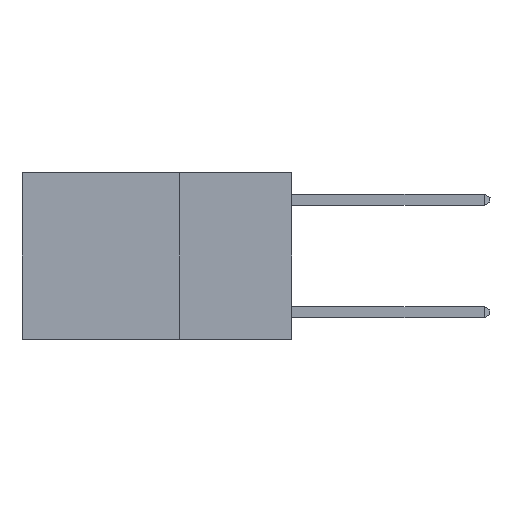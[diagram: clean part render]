
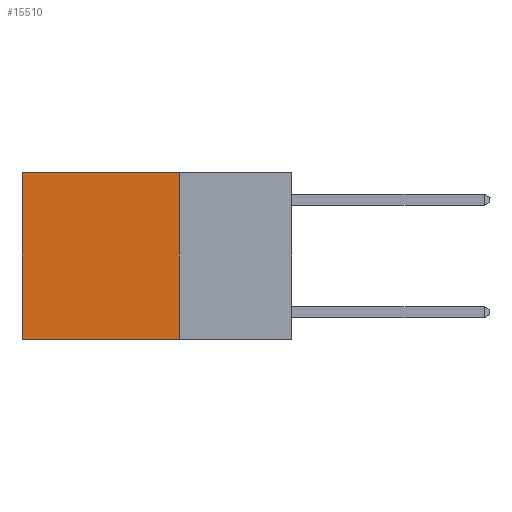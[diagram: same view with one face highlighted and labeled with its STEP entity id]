
A CAD part, left-side view. The second image highlights one B-rep face of the part: STEP entity #15510.
In plain terms, the highlighted planar face has unit normal (-1, 0, 0).
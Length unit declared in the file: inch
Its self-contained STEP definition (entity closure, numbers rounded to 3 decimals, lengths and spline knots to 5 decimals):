
#1141 = VECTOR ( 'NONE', #3060, 39.37008 ) ;
#2734 = CARTESIAN_POINT ( 'NONE',  ( 0.2625, 0.25, 0. ) ) ;
#3060 = DIRECTION ( 'NONE',  ( 0., 0., -1. ) ) ;
#3104 = ORIENTED_EDGE ( 'NONE', *, *, #19769, .T. ) ;
#3151 = CARTESIAN_POINT ( 'NONE',  ( 0.2625, 0.6, 0. ) ) ;
#4069 = CARTESIAN_POINT ( 'NONE',  ( 0.2625, 0.6, -0.37 ) ) ;
#4252 = VERTEX_POINT ( 'NONE', #4069 ) ;
#4399 = CARTESIAN_POINT ( 'NONE',  ( 0.2625, 0.6, 0. ) ) ;
#5651 = DIRECTION ( 'NONE',  ( 0., 1., 0. ) ) ;
#5827 = VERTEX_POINT ( 'NONE', #9938 ) ;
#6023 = LINE ( 'NONE', #2734, #1141 ) ;
#6456 = AXIS2_PLACEMENT_3D ( 'NONE', #19977, #14849, #18437 ) ;
#7572 = CARTESIAN_POINT ( 'NONE',  ( 0.2625, 0.25, 0. ) ) ;
#7703 = PLANE ( 'NONE',  #6456 ) ;
#7968 = VECTOR ( 'NONE', #11126, 39.37008 ) ;
#7991 = VERTEX_POINT ( 'NONE', #3151 ) ;
#8322 = VECTOR ( 'NONE', #20836, 39.37008 ) ;
#8337 = VERTEX_POINT ( 'NONE', #12526 ) ;
#9184 = ORIENTED_EDGE ( 'NONE', *, *, #11539, .F. ) ;
#9245 = LINE ( 'NONE', #7572, #8322 ) ;
#9938 = CARTESIAN_POINT ( 'NONE',  ( 0.2625, 0.25, -0.37 ) ) ;
#11126 = DIRECTION ( 'NONE',  ( 0., 0., -1. ) ) ;
#11258 = FACE_OUTER_BOUND ( 'NONE', #11739, .T. ) ;
#11539 = EDGE_CURVE ( 'NONE', #8337, #5827, #6023, .T. ) ;
#11739 = EDGE_LOOP ( 'NONE', ( #3104, #16492, #9184, #18094 ) ) ;
#12526 = CARTESIAN_POINT ( 'NONE',  ( 0.2625, 0.25, 0. ) ) ;
#14849 = DIRECTION ( 'NONE',  ( 1., 0., 0. ) ) ;
#14915 = EDGE_CURVE ( 'NONE', #5827, #4252, #15749, .T. ) ;
#15510 = ADVANCED_FACE ( 'NONE', ( #11258 ), #7703, .F. ) ;
#15749 = LINE ( 'NONE', #19235, #18399 ) ;
#16038 = LINE ( 'NONE', #4399, #7968 ) ;
#16492 = ORIENTED_EDGE ( 'NONE', *, *, #14915, .F. ) ;
#18094 = ORIENTED_EDGE ( 'NONE', *, *, #19739, .T. ) ;
#18399 = VECTOR ( 'NONE', #5651, 39.37008 ) ;
#18437 = DIRECTION ( 'NONE',  ( 0., 0., -1. ) ) ;
#19235 = CARTESIAN_POINT ( 'NONE',  ( 0.2625, 0.25, -0.37 ) ) ;
#19739 = EDGE_CURVE ( 'NONE', #8337, #7991, #9245, .T. ) ;
#19769 = EDGE_CURVE ( 'NONE', #7991, #4252, #16038, .T. ) ;
#19977 = CARTESIAN_POINT ( 'NONE',  ( 0.2625, 0.25, 0. ) ) ;
#20836 = DIRECTION ( 'NONE',  ( 0., 1., 0. ) ) ;
